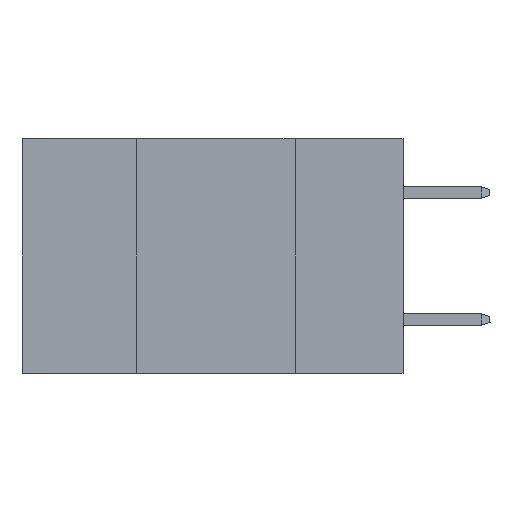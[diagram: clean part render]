
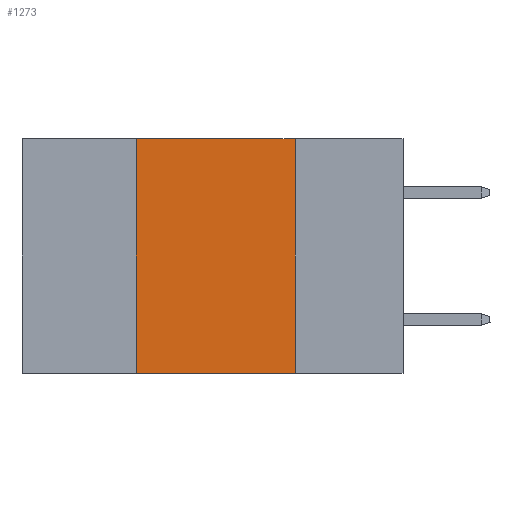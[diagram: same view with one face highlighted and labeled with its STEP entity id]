
A CAD part, left-side view. The second image highlights one B-rep face of the part: STEP entity #1273.
In plain terms, the highlighted planar face has unit normal (-1, 0, 0).
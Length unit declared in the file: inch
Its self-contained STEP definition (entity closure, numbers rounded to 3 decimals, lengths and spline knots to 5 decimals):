
#319 = ORIENTED_EDGE ( 'NONE', *, *, #9359, .F. ) ;
#800 = VECTOR ( 'NONE', #15112, 39.37008 ) ;
#1148 = DIRECTION ( 'NONE',  ( 0., 0., -1. ) ) ;
#1273 = ADVANCED_FACE ( 'NONE', ( #14308 ), #2721, .F. ) ;
#1406 = LINE ( 'NONE', #3487, #14209 ) ;
#1678 = ORIENTED_EDGE ( 'NONE', *, *, #5629, .F. ) ;
#2721 = PLANE ( 'NONE',  #3461 ) ;
#2916 = EDGE_LOOP ( 'NONE', ( #319, #1678, #11445, #17161 ) ) ;
#3005 = VERTEX_POINT ( 'NONE', #3705 ) ;
#3293 = VERTEX_POINT ( 'NONE', #9782 ) ;
#3348 = DIRECTION ( 'NONE',  ( 0., 0., -1. ) ) ;
#3461 = AXIS2_PLACEMENT_3D ( 'NONE', #5879, #7465, #1148 ) ;
#3487 = CARTESIAN_POINT ( 'NONE',  ( 0., 0.42, 0. ) ) ;
#3705 = CARTESIAN_POINT ( 'NONE',  ( 0., 0.42, 0. ) ) ;
#4070 = VECTOR ( 'NONE', #11415, 39.37008 ) ;
#4248 = EDGE_CURVE ( 'NONE', #3293, #3005, #1406, .T. ) ;
#4981 = CARTESIAN_POINT ( 'NONE',  ( 0., 0.6, -0.37 ) ) ;
#5629 = EDGE_CURVE ( 'NONE', #3005, #19369, #7100, .T. ) ;
#5879 = CARTESIAN_POINT ( 'NONE',  ( 0., 0.6, 0. ) ) ;
#6226 = CARTESIAN_POINT ( 'NONE',  ( 0., 0.17, 0. ) ) ;
#7100 = LINE ( 'NONE', #8685, #800 ) ;
#7465 = DIRECTION ( 'NONE',  ( 1., 0., 0. ) ) ;
#8341 = LINE ( 'NONE', #4981, #4070 ) ;
#8685 = CARTESIAN_POINT ( 'NONE',  ( 0., 0.6, 0. ) ) ;
#9056 = EDGE_CURVE ( 'NONE', #3293, #19004, #8341, .T. ) ;
#9359 = EDGE_CURVE ( 'NONE', #19369, #19004, #19476, .T. ) ;
#9782 = CARTESIAN_POINT ( 'NONE',  ( 0., 0.42, -0.37 ) ) ;
#11415 = DIRECTION ( 'NONE',  ( 0., -1., 0. ) ) ;
#11445 = ORIENTED_EDGE ( 'NONE', *, *, #4248, .F. ) ;
#13506 = VECTOR ( 'NONE', #3348, 39.37008 ) ;
#14209 = VECTOR ( 'NONE', #19121, 39.37008 ) ;
#14290 = CARTESIAN_POINT ( 'NONE',  ( 0., 0.17, -0.37 ) ) ;
#14308 = FACE_OUTER_BOUND ( 'NONE', #2916, .T. ) ;
#15112 = DIRECTION ( 'NONE',  ( 0., -1., 0. ) ) ;
#17161 = ORIENTED_EDGE ( 'NONE', *, *, #9056, .T. ) ;
#19004 = VERTEX_POINT ( 'NONE', #14290 ) ;
#19121 = DIRECTION ( 'NONE',  ( 0., 0., 1. ) ) ;
#19369 = VERTEX_POINT ( 'NONE', #20709 ) ;
#19476 = LINE ( 'NONE', #6226, #13506 ) ;
#20709 = CARTESIAN_POINT ( 'NONE',  ( 0., 0.17, 0. ) ) ;
